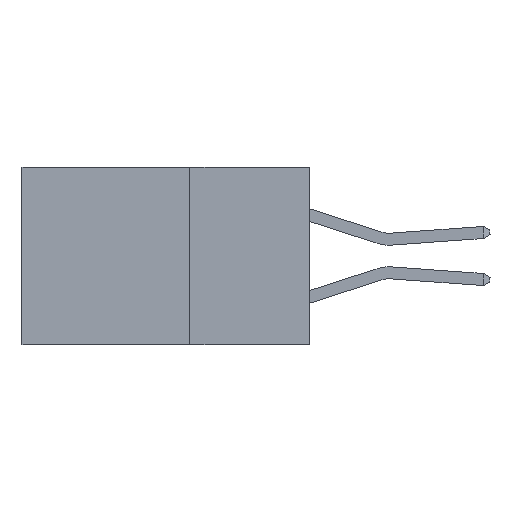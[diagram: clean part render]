
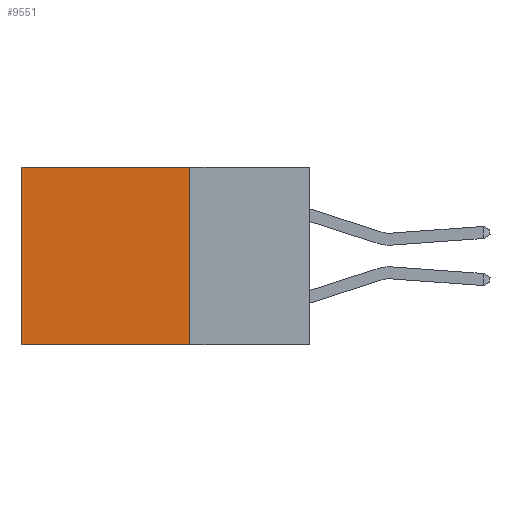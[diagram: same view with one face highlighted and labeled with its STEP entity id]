
A CAD part, left-side view. The second image highlights one B-rep face of the part: STEP entity #9551.
In plain terms, the highlighted planar face has unit normal (-1, 0, 0).
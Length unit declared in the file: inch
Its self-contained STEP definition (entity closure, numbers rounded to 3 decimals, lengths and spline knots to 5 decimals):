
#205 = EDGE_CURVE ( 'NONE', #5936, #8417, #12000, .T. ) ;
#469 = CARTESIAN_POINT ( 'NONE',  ( 0.298, 0.25, -0.37 ) ) ;
#763 = EDGE_CURVE ( 'NONE', #11270, #8417, #5403, .T. ) ;
#1062 = CARTESIAN_POINT ( 'NONE',  ( 0.298, 0.25, 0. ) ) ;
#1592 = VERTEX_POINT ( 'NONE', #8224 ) ;
#2081 = CARTESIAN_POINT ( 'NONE',  ( 0.298, 0.25, 0. ) ) ;
#2266 = LINE ( 'NONE', #1062, #11544 ) ;
#2678 = FACE_OUTER_BOUND ( 'NONE', #12484, .T. ) ;
#2952 = ORIENTED_EDGE ( 'NONE', *, *, #8163, .F. ) ;
#3971 = VECTOR ( 'NONE', #4555, 39.37008 ) ;
#4240 = DIRECTION ( 'NONE',  ( 1., 0., 0. ) ) ;
#4555 = DIRECTION ( 'NONE',  ( 0., 1., 0. ) ) ;
#4762 = VECTOR ( 'NONE', #12275, 39.37008 ) ;
#4997 = AXIS2_PLACEMENT_3D ( 'NONE', #11331, #4240, #7288 ) ;
#5262 = PLANE ( 'NONE',  #4997 ) ;
#5403 = LINE ( 'NONE', #469, #3971 ) ;
#5936 = VERTEX_POINT ( 'NONE', #9290 ) ;
#7288 = DIRECTION ( 'NONE',  ( 0., 0., -1. ) ) ;
#7324 = LINE ( 'NONE', #2081, #13081 ) ;
#8163 = EDGE_CURVE ( 'NONE', #1592, #11270, #2266, .T. ) ;
#8224 = CARTESIAN_POINT ( 'NONE',  ( 0.298, 0.25, 0. ) ) ;
#8417 = VERTEX_POINT ( 'NONE', #9755 ) ;
#8550 = ORIENTED_EDGE ( 'NONE', *, *, #763, .F. ) ;
#8684 = CARTESIAN_POINT ( 'NONE',  ( 0.298, 0.25, -0.37 ) ) ;
#9239 = DIRECTION ( 'NONE',  ( 0., 1., 0. ) ) ;
#9290 = CARTESIAN_POINT ( 'NONE',  ( 0.298, 0.6, 0. ) ) ;
#9551 = ADVANCED_FACE ( 'NONE', ( #2678 ), #5262, .F. ) ;
#9670 = EDGE_CURVE ( 'NONE', #1592, #5936, #7324, .T. ) ;
#9755 = CARTESIAN_POINT ( 'NONE',  ( 0.298, 0.6, -0.37 ) ) ;
#11140 = DIRECTION ( 'NONE',  ( 0., 0., -1. ) ) ;
#11270 = VERTEX_POINT ( 'NONE', #8684 ) ;
#11331 = CARTESIAN_POINT ( 'NONE',  ( 0.298, 0.25, 0. ) ) ;
#11459 = ORIENTED_EDGE ( 'NONE', *, *, #205, .T. ) ;
#11544 = VECTOR ( 'NONE', #11140, 39.37008 ) ;
#12000 = LINE ( 'NONE', #12362, #4762 ) ;
#12275 = DIRECTION ( 'NONE',  ( 0., 0., -1. ) ) ;
#12362 = CARTESIAN_POINT ( 'NONE',  ( 0.298, 0.6, 0. ) ) ;
#12484 = EDGE_LOOP ( 'NONE', ( #11459, #8550, #2952, #12939 ) ) ;
#12939 = ORIENTED_EDGE ( 'NONE', *, *, #9670, .T. ) ;
#13081 = VECTOR ( 'NONE', #9239, 39.37008 ) ;
